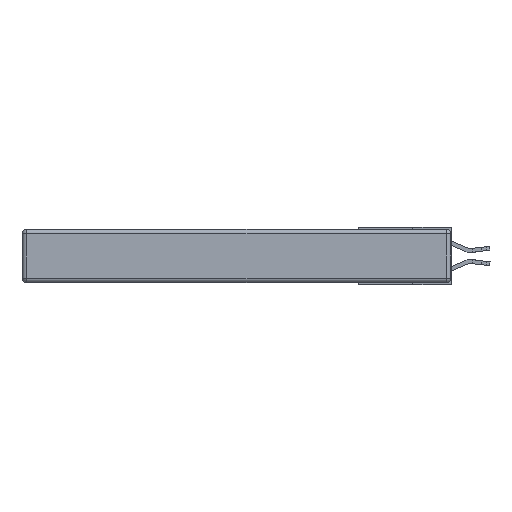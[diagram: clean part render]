
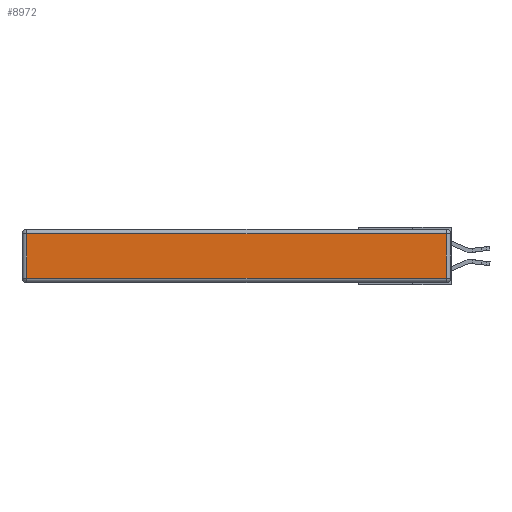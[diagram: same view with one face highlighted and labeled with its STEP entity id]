
A CAD part, left-side view. The second image highlights one B-rep face of the part: STEP entity #8972.
In plain terms, the highlighted planar face has unit normal (-1, 0, 0).
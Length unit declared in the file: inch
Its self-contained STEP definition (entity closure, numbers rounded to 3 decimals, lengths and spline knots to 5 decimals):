
#999 = CARTESIAN_POINT ( 'NONE',  ( 0., 0., -0.313 ) ) ;
#1124 = LINE ( 'NONE', #4937, #11678 ) ;
#1128 = EDGE_CURVE ( 'NONE', #26514, #20922, #1526, .T. ) ;
#1526 = LINE ( 'NONE', #11318, #24654 ) ;
#1925 = EDGE_CURVE ( 'NONE', #14604, #24067, #1124, .T. ) ;
#2060 = ORIENTED_EDGE ( 'NONE', *, *, #1128, .T. ) ;
#4317 = EDGE_LOOP ( 'NONE', ( #8395, #11042, #11454, #2060 ) ) ;
#4517 = LINE ( 'NONE', #22454, #27560 ) ;
#4937 = CARTESIAN_POINT ( 'NONE',  ( 0., 0.03, -0.343 ) ) ;
#7072 = CARTESIAN_POINT ( 'NONE',  ( 0., 2.72, -0.313 ) ) ;
#7331 = DIRECTION ( 'NONE',  ( -1., 0., 0. ) ) ;
#8235 = CARTESIAN_POINT ( 'NONE',  ( 0., 0.03, -0.03 ) ) ;
#8395 = ORIENTED_EDGE ( 'NONE', *, *, #16963, .T. ) ;
#8972 = ADVANCED_FACE ( 'NONE', ( #16177 ), #23022, .T. ) ;
#9805 = LINE ( 'NONE', #999, #17721 ) ;
#11042 = ORIENTED_EDGE ( 'NONE', *, *, #1925, .T. ) ;
#11318 = CARTESIAN_POINT ( 'NONE',  ( 0., 2.72, -0.343 ) ) ;
#11454 = ORIENTED_EDGE ( 'NONE', *, *, #27477, .T. ) ;
#11678 = VECTOR ( 'NONE', #25560, 39.37008 ) ;
#14604 = VERTEX_POINT ( 'NONE', #15486 ) ;
#15372 = AXIS2_PLACEMENT_3D ( 'NONE', #18517, #7331, #23321 ) ;
#15486 = CARTESIAN_POINT ( 'NONE',  ( 0., 0.03, -0.313 ) ) ;
#15512 = DIRECTION ( 'NONE',  ( 0., 0., -1. ) ) ;
#16177 = FACE_OUTER_BOUND ( 'NONE', #4317, .T. ) ;
#16723 = CARTESIAN_POINT ( 'NONE',  ( 0., 2.72, -0.03 ) ) ;
#16963 = EDGE_CURVE ( 'NONE', #20922, #14604, #9805, .T. ) ;
#17721 = VECTOR ( 'NONE', #19514, 39.37008 ) ;
#17937 = DIRECTION ( 'NONE',  ( 0., 1., 0. ) ) ;
#18517 = CARTESIAN_POINT ( 'NONE',  ( 0., 0., -0.343 ) ) ;
#19514 = DIRECTION ( 'NONE',  ( 0., -1., 0. ) ) ;
#20922 = VERTEX_POINT ( 'NONE', #7072 ) ;
#22454 = CARTESIAN_POINT ( 'NONE',  ( 0., 2.75, -0.03 ) ) ;
#23022 = PLANE ( 'NONE',  #15372 ) ;
#23321 = DIRECTION ( 'NONE',  ( 0., 0., 1. ) ) ;
#24067 = VERTEX_POINT ( 'NONE', #8235 ) ;
#24654 = VECTOR ( 'NONE', #15512, 39.37008 ) ;
#25560 = DIRECTION ( 'NONE',  ( 0., 0., 1. ) ) ;
#26514 = VERTEX_POINT ( 'NONE', #16723 ) ;
#27477 = EDGE_CURVE ( 'NONE', #24067, #26514, #4517, .T. ) ;
#27560 = VECTOR ( 'NONE', #17937, 39.37008 ) ;
